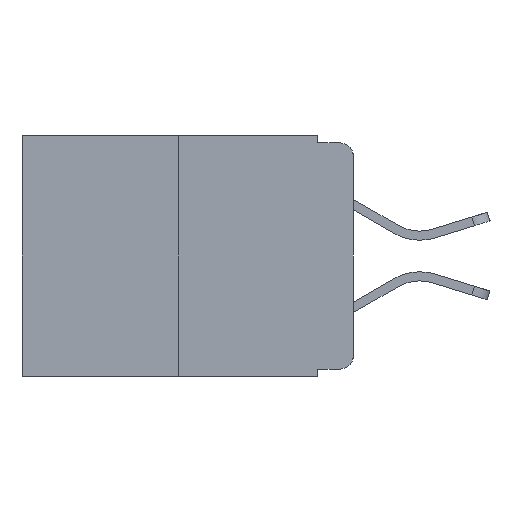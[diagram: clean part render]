
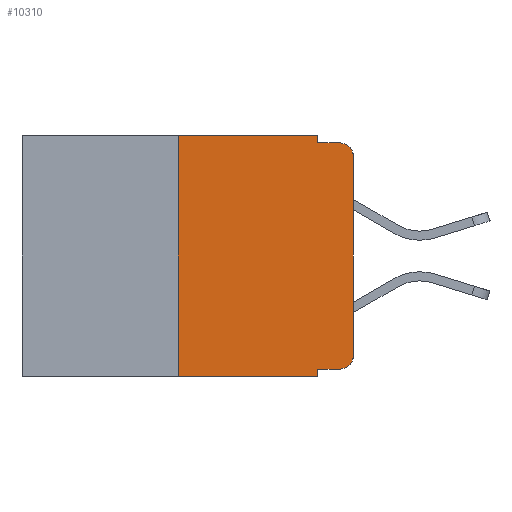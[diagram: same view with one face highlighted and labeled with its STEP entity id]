
A CAD part, left-side view. The second image highlights one B-rep face of the part: STEP entity #10310.
In plain terms, the highlighted planar face has unit normal (-1, 0, 0).
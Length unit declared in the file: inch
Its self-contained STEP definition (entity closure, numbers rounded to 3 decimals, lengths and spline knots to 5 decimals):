
#105 = ORIENTED_EDGE ( 'NONE', *, *, #228, .T. ) ;
#228 = EDGE_CURVE ( 'NONE', #11077, #12721, #9788, .T. ) ;
#806 = CARTESIAN_POINT ( 'NONE',  ( 0., 0.25, -0.343 ) ) ;
#842 = EDGE_CURVE ( 'NONE', #14586, #10474, #5140, .T. ) ;
#892 = ORIENTED_EDGE ( 'NONE', *, *, #12089, .F. ) ;
#1181 = EDGE_CURVE ( 'NONE', #11091, #13179, #8568, .T. ) ;
#1361 = CIRCLE ( 'NONE', #5040, 0.02 ) ;
#1450 = DIRECTION ( 'NONE',  ( 0., 0., -1. ) ) ;
#1644 = CARTESIAN_POINT ( 'NONE',  ( 0., 0.02, -0.333 ) ) ;
#1648 = CARTESIAN_POINT ( 'NONE',  ( 0., 0.02, -0.03 ) ) ;
#1714 = DIRECTION ( 'NONE',  ( 0., 0., 1. ) ) ;
#2026 = CARTESIAN_POINT ( 'NONE',  ( 0., 0.02, -0.01 ) ) ;
#2161 = DIRECTION ( 'NONE',  ( 0., 0., -1. ) ) ;
#2238 = VECTOR ( 'NONE', #5970, 39.37008 ) ;
#2362 = DIRECTION ( 'NONE',  ( 0., 0., 1. ) ) ;
#2433 = VERTEX_POINT ( 'NONE', #1644 ) ;
#2788 = ORIENTED_EDGE ( 'NONE', *, *, #16021, .F. ) ;
#3382 = VECTOR ( 'NONE', #2362, 39.37008 ) ;
#3745 = VECTOR ( 'NONE', #1714, 39.37008 ) ;
#3987 = CARTESIAN_POINT ( 'NONE',  ( 0., 0.25, 0. ) ) ;
#4042 = DIRECTION ( 'NONE',  ( -1., 0., 0. ) ) ;
#4466 = CARTESIAN_POINT ( 'NONE',  ( 0., 0., 0. ) ) ;
#4563 = CARTESIAN_POINT ( 'NONE',  ( 0., 0.473, 0. ) ) ;
#4952 = CARTESIAN_POINT ( 'NONE',  ( 0., 0.02, -0.313 ) ) ;
#5040 = AXIS2_PLACEMENT_3D ( 'NONE', #4952, #13100, #11776 ) ;
#5140 = LINE ( 'NONE', #15942, #6716 ) ;
#5580 = EDGE_CURVE ( 'NONE', #16482, #11077, #16605, .T. ) ;
#5632 = FACE_OUTER_BOUND ( 'NONE', #7800, .T. ) ;
#5949 = VERTEX_POINT ( 'NONE', #8510 ) ;
#5970 = DIRECTION ( 'NONE',  ( 0., -1., 0. ) ) ;
#6312 = ORIENTED_EDGE ( 'NONE', *, *, #5580, .T. ) ;
#6394 = AXIS2_PLACEMENT_3D ( 'NONE', #1648, #4042, #16453 ) ;
#6605 = CARTESIAN_POINT ( 'NONE',  ( 0., 0.25, 0. ) ) ;
#6716 = VECTOR ( 'NONE', #7875, 39.37008 ) ;
#6837 = ORIENTED_EDGE ( 'NONE', *, *, #842, .T. ) ;
#7676 = LINE ( 'NONE', #8988, #14711 ) ;
#7773 = VERTEX_POINT ( 'NONE', #16843 ) ;
#7800 = EDGE_LOOP ( 'NONE', ( #6312, #105, #16014, #2788, #15361, #11795, #6837, #892, #10883, #9477 ) ) ;
#7875 = DIRECTION ( 'NONE',  ( 0., -1., 0. ) ) ;
#8510 = CARTESIAN_POINT ( 'NONE',  ( 0., 0.051, -0.01 ) ) ;
#8568 = LINE ( 'NONE', #12913, #14351 ) ;
#8815 = DIRECTION ( 'NONE',  ( 0., -1., 0. ) ) ;
#8988 = CARTESIAN_POINT ( 'NONE',  ( 0., 0.051, -0.01 ) ) ;
#9477 = ORIENTED_EDGE ( 'NONE', *, *, #9545, .T. ) ;
#9545 = EDGE_CURVE ( 'NONE', #2433, #16482, #1361, .T. ) ;
#9788 = CIRCLE ( 'NONE', #6394, 0.02 ) ;
#9955 = DIRECTION ( 'NONE',  ( 1., 0., 0. ) ) ;
#10310 = ADVANCED_FACE ( 'NONE', ( #5632 ), #12540, .F. ) ;
#10316 = LINE ( 'NONE', #14290, #11677 ) ;
#10430 = EDGE_CURVE ( 'NONE', #7773, #2433, #17035, .T. ) ;
#10474 = VERTEX_POINT ( 'NONE', #17137 ) ;
#10883 = ORIENTED_EDGE ( 'NONE', *, *, #10430, .T. ) ;
#11077 = VERTEX_POINT ( 'NONE', #16041 ) ;
#11091 = VERTEX_POINT ( 'NONE', #3987 ) ;
#11677 = VECTOR ( 'NONE', #2161, 39.37008 ) ;
#11776 = DIRECTION ( 'NONE',  ( 0., 0., -1. ) ) ;
#11795 = ORIENTED_EDGE ( 'NONE', *, *, #13243, .F. ) ;
#11935 = DIRECTION ( 'NONE',  ( 0., -1., 0. ) ) ;
#12089 = EDGE_CURVE ( 'NONE', #7773, #10474, #16674, .T. ) ;
#12200 = VECTOR ( 'NONE', #1450, 39.37008 ) ;
#12284 = DIRECTION ( 'NONE',  ( 0., 0., -1. ) ) ;
#12540 = PLANE ( 'NONE',  #17524 ) ;
#12619 = CARTESIAN_POINT ( 'NONE',  ( 0., 0.051, 0. ) ) ;
#12721 = VERTEX_POINT ( 'NONE', #2026 ) ;
#12913 = CARTESIAN_POINT ( 'NONE',  ( 0., 0.473, 0. ) ) ;
#12965 = CARTESIAN_POINT ( 'NONE',  ( 0., 0.051, -0.333 ) ) ;
#13100 = DIRECTION ( 'NONE',  ( -1., 0., 0. ) ) ;
#13179 = VERTEX_POINT ( 'NONE', #14221 ) ;
#13227 = EDGE_CURVE ( 'NONE', #5949, #12721, #7676, .T. ) ;
#13243 = EDGE_CURVE ( 'NONE', #14586, #11091, #14396, .T. ) ;
#13388 = CARTESIAN_POINT ( 'NONE',  ( 0., 0., -0.313 ) ) ;
#14221 = CARTESIAN_POINT ( 'NONE',  ( 0., 0.051, 0. ) ) ;
#14290 = CARTESIAN_POINT ( 'NONE',  ( 0., 0.051, 0. ) ) ;
#14351 = VECTOR ( 'NONE', #8815, 39.37008 ) ;
#14396 = LINE ( 'NONE', #6605, #3382 ) ;
#14586 = VERTEX_POINT ( 'NONE', #806 ) ;
#14711 = VECTOR ( 'NONE', #11935, 39.37008 ) ;
#15361 = ORIENTED_EDGE ( 'NONE', *, *, #1181, .F. ) ;
#15942 = CARTESIAN_POINT ( 'NONE',  ( 0., 0.473, -0.343 ) ) ;
#16014 = ORIENTED_EDGE ( 'NONE', *, *, #13227, .F. ) ;
#16021 = EDGE_CURVE ( 'NONE', #13179, #5949, #10316, .T. ) ;
#16041 = CARTESIAN_POINT ( 'NONE',  ( 0., 0., -0.03 ) ) ;
#16453 = DIRECTION ( 'NONE',  ( 0., 0., -1. ) ) ;
#16482 = VERTEX_POINT ( 'NONE', #13388 ) ;
#16605 = LINE ( 'NONE', #4466, #3745 ) ;
#16674 = LINE ( 'NONE', #12619, #12200 ) ;
#16843 = CARTESIAN_POINT ( 'NONE',  ( 0., 0.051, -0.333 ) ) ;
#17035 = LINE ( 'NONE', #12965, #2238 ) ;
#17137 = CARTESIAN_POINT ( 'NONE',  ( 0., 0.051, -0.343 ) ) ;
#17524 = AXIS2_PLACEMENT_3D ( 'NONE', #4563, #9955, #12284 ) ;
